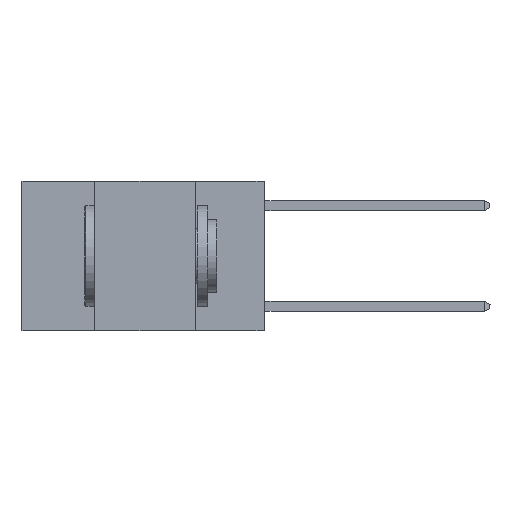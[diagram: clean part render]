
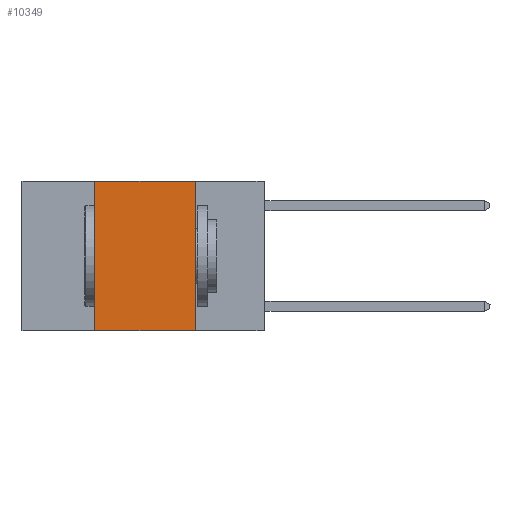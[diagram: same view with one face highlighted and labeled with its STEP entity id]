
A CAD part, left-side view. The second image highlights one B-rep face of the part: STEP entity #10349.
In plain terms, the highlighted planar face has unit normal (-1, 0, 0).
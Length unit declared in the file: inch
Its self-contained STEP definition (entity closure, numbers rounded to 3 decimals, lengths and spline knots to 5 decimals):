
#316 = DIRECTION ( 'NONE',  ( 0., 0., -1. ) ) ;
#823 = VERTEX_POINT ( 'NONE', #14634 ) ;
#973 = EDGE_CURVE ( 'NONE', #10732, #15167, #14428, .T. ) ;
#1750 = VERTEX_POINT ( 'NONE', #11490 ) ;
#2051 = EDGE_CURVE ( 'NONE', #1750, #823, #9862, .T. ) ;
#2188 = CARTESIAN_POINT ( 'NONE',  ( 0., 0.42, 0. ) ) ;
#2542 = CARTESIAN_POINT ( 'NONE',  ( 0., 0.17, 0. ) ) ;
#5336 = DIRECTION ( 'NONE',  ( 0., -1., 0. ) ) ;
#5755 = CARTESIAN_POINT ( 'NONE',  ( 0., 0.6, 0. ) ) ;
#6841 = DIRECTION ( 'NONE',  ( 0., 0., -1. ) ) ;
#9862 = LINE ( 'NONE', #18426, #20668 ) ;
#10231 = ORIENTED_EDGE ( 'NONE', *, *, #18312, .F. ) ;
#10349 = ADVANCED_FACE ( 'NONE', ( #19710 ), #22952, .F. ) ;
#10576 = ORIENTED_EDGE ( 'NONE', *, *, #11513, .F. ) ;
#10732 = VERTEX_POINT ( 'NONE', #20434 ) ;
#11490 = CARTESIAN_POINT ( 'NONE',  ( 0., 0.42, -0.37 ) ) ;
#11513 = EDGE_CURVE ( 'NONE', #1750, #10732, #13947, .T. ) ;
#11699 = EDGE_LOOP ( 'NONE', ( #10231, #18857, #10576, #11871 ) ) ;
#11871 = ORIENTED_EDGE ( 'NONE', *, *, #2051, .T. ) ;
#12895 = DIRECTION ( 'NONE',  ( 1., 0., 0. ) ) ;
#13781 = VECTOR ( 'NONE', #6841, 39.37008 ) ;
#13947 = LINE ( 'NONE', #2188, #19336 ) ;
#14428 = LINE ( 'NONE', #5755, #25204 ) ;
#14634 = CARTESIAN_POINT ( 'NONE',  ( 0., 0.17, -0.37 ) ) ;
#15167 = VERTEX_POINT ( 'NONE', #20456 ) ;
#18312 = EDGE_CURVE ( 'NONE', #15167, #823, #24530, .T. ) ;
#18389 = DIRECTION ( 'NONE',  ( 0., -1., 0. ) ) ;
#18426 = CARTESIAN_POINT ( 'NONE',  ( 0., 0.6, -0.37 ) ) ;
#18857 = ORIENTED_EDGE ( 'NONE', *, *, #973, .F. ) ;
#19336 = VECTOR ( 'NONE', #24782, 39.37008 ) ;
#19390 = AXIS2_PLACEMENT_3D ( 'NONE', #25015, #12895, #316 ) ;
#19710 = FACE_OUTER_BOUND ( 'NONE', #11699, .T. ) ;
#20434 = CARTESIAN_POINT ( 'NONE',  ( 0., 0.42, 0. ) ) ;
#20456 = CARTESIAN_POINT ( 'NONE',  ( 0., 0.17, 0. ) ) ;
#20668 = VECTOR ( 'NONE', #18389, 39.37008 ) ;
#22952 = PLANE ( 'NONE',  #19390 ) ;
#24530 = LINE ( 'NONE', #2542, #13781 ) ;
#24782 = DIRECTION ( 'NONE',  ( 0., 0., 1. ) ) ;
#25015 = CARTESIAN_POINT ( 'NONE',  ( 0., 0.6, 0. ) ) ;
#25204 = VECTOR ( 'NONE', #5336, 39.37008 ) ;
